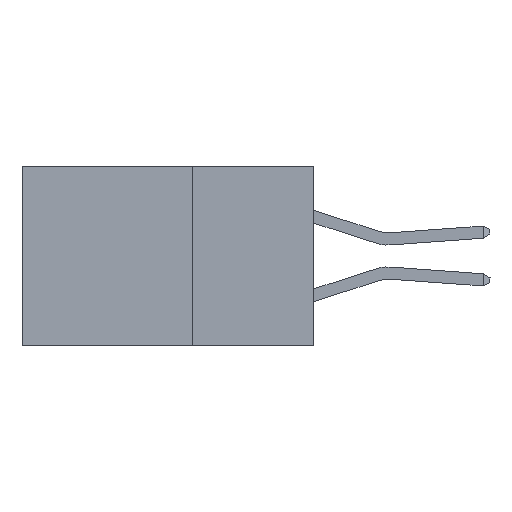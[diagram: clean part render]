
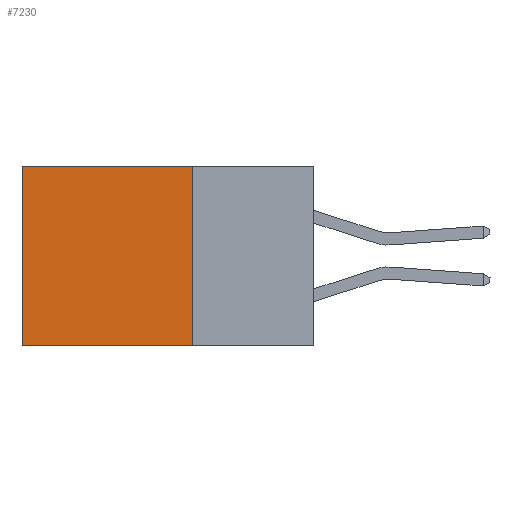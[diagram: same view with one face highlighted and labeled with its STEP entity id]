
A CAD part, left-side view. The second image highlights one B-rep face of the part: STEP entity #7230.
In plain terms, the highlighted planar face has unit normal (-1, 0, 0).
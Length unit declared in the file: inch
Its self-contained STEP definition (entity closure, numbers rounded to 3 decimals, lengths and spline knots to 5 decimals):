
#129 = CARTESIAN_POINT ( 'NONE',  ( 0.2875, 0.25, 0. ) ) ;
#362 = LINE ( 'NONE', #21676, #5849 ) ;
#509 = LINE ( 'NONE', #5546, #11005 ) ;
#1784 = ORIENTED_EDGE ( 'NONE', *, *, #10838, .T. ) ;
#2753 = CARTESIAN_POINT ( 'NONE',  ( 0.2875, 0.6, -0.37 ) ) ;
#4129 = DIRECTION ( 'NONE',  ( 0., 0., -1. ) ) ;
#4591 = EDGE_LOOP ( 'NONE', ( #21598, #22920, #11159, #1784 ) ) ;
#5455 = DIRECTION ( 'NONE',  ( 0., 1., 0. ) ) ;
#5546 = CARTESIAN_POINT ( 'NONE',  ( 0.2875, 0.25, -0.37 ) ) ;
#5826 = LINE ( 'NONE', #8745, #7264 ) ;
#5849 = VECTOR ( 'NONE', #12877, 39.37008 ) ;
#6666 = CARTESIAN_POINT ( 'NONE',  ( 0.2875, 0.25, 0. ) ) ;
#6765 = DIRECTION ( 'NONE',  ( 0., 0., -1. ) ) ;
#7230 = ADVANCED_FACE ( 'NONE', ( #25535 ), #18029, .F. ) ;
#7264 = VECTOR ( 'NONE', #4129, 39.37008 ) ;
#8745 = CARTESIAN_POINT ( 'NONE',  ( 0.2875, 0.6, 0. ) ) ;
#9804 = EDGE_CURVE ( 'NONE', #22308, #28934, #28860, .T. ) ;
#9805 = VERTEX_POINT ( 'NONE', #13996 ) ;
#10838 = EDGE_CURVE ( 'NONE', #22308, #9805, #362, .T. ) ;
#10930 = EDGE_CURVE ( 'NONE', #9805, #28171, #5826, .T. ) ;
#11005 = VECTOR ( 'NONE', #5455, 39.37008 ) ;
#11159 = ORIENTED_EDGE ( 'NONE', *, *, #9804, .F. ) ;
#12355 = AXIS2_PLACEMENT_3D ( 'NONE', #6666, #27281, #6765 ) ;
#12877 = DIRECTION ( 'NONE',  ( 0., 1., 0. ) ) ;
#13740 = VECTOR ( 'NONE', #16300, 39.37008 ) ;
#13996 = CARTESIAN_POINT ( 'NONE',  ( 0.2875, 0.6, 0. ) ) ;
#15201 = CARTESIAN_POINT ( 'NONE',  ( 0.2875, 0.25, -0.37 ) ) ;
#16300 = DIRECTION ( 'NONE',  ( 0., 0., -1. ) ) ;
#18029 = PLANE ( 'NONE',  #12355 ) ;
#19016 = EDGE_CURVE ( 'NONE', #28934, #28171, #509, .T. ) ;
#20880 = CARTESIAN_POINT ( 'NONE',  ( 0.2875, 0.25, 0. ) ) ;
#21598 = ORIENTED_EDGE ( 'NONE', *, *, #10930, .T. ) ;
#21676 = CARTESIAN_POINT ( 'NONE',  ( 0.2875, 0.25, 0. ) ) ;
#22308 = VERTEX_POINT ( 'NONE', #129 ) ;
#22920 = ORIENTED_EDGE ( 'NONE', *, *, #19016, .F. ) ;
#25535 = FACE_OUTER_BOUND ( 'NONE', #4591, .T. ) ;
#27281 = DIRECTION ( 'NONE',  ( 1., 0., 0. ) ) ;
#28171 = VERTEX_POINT ( 'NONE', #2753 ) ;
#28860 = LINE ( 'NONE', #20880, #13740 ) ;
#28934 = VERTEX_POINT ( 'NONE', #15201 ) ;
